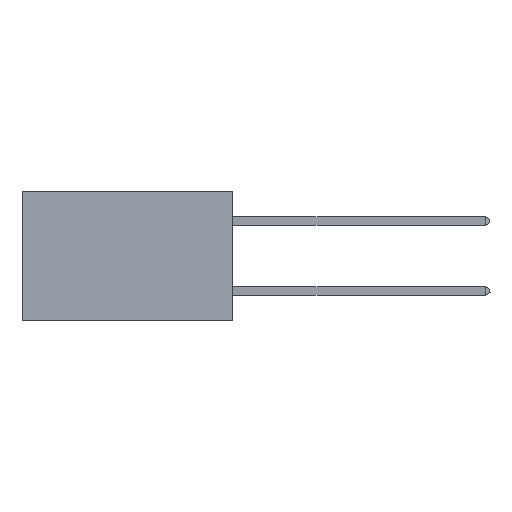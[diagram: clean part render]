
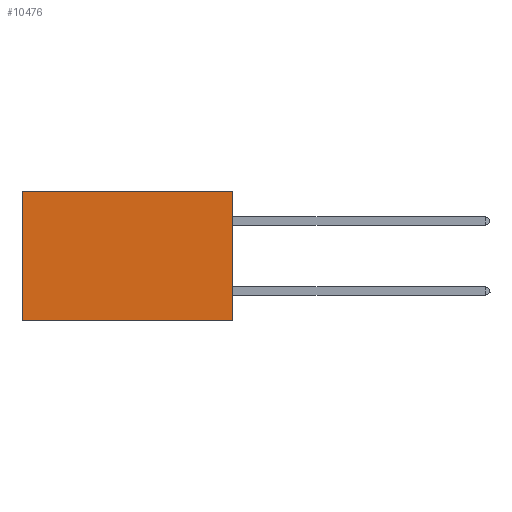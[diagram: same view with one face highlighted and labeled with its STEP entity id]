
A CAD part, left-side view. The second image highlights one B-rep face of the part: STEP entity #10476.
In plain terms, the highlighted planar face has unit normal (-1, 0, 0).
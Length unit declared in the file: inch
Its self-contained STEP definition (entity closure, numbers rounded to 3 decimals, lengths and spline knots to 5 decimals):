
#1293 = VERTEX_POINT ( 'NONE', #9393 ) ;
#2304 = LINE ( 'NONE', #4347, #10646 ) ;
#3001 = EDGE_LOOP ( 'NONE', ( #9604, #19115, #9697, #12411 ) ) ;
#3123 = LINE ( 'NONE', #4594, #8878 ) ;
#3323 = EDGE_CURVE ( 'NONE', #1293, #5030, #2304, .T. ) ;
#4347 = CARTESIAN_POINT ( 'NONE',  ( 0.2875, 0.6, 0. ) ) ;
#4439 = AXIS2_PLACEMENT_3D ( 'NONE', #18264, #18469, #19945 ) ;
#4594 = CARTESIAN_POINT ( 'NONE',  ( 0.2875, 0., 0. ) ) ;
#4647 = VERTEX_POINT ( 'NONE', #18371 ) ;
#5030 = VERTEX_POINT ( 'NONE', #10223 ) ;
#6122 = VECTOR ( 'NONE', #7002, 39.37008 ) ;
#6576 = PLANE ( 'NONE',  #4439 ) ;
#7002 = DIRECTION ( 'NONE',  ( 0., 1., 0. ) ) ;
#7457 = LINE ( 'NONE', #11922, #6122 ) ;
#8878 = VECTOR ( 'NONE', #21415, 39.37008 ) ;
#9393 = CARTESIAN_POINT ( 'NONE',  ( 0.2875, 0.6, 0. ) ) ;
#9483 = DIRECTION ( 'NONE',  ( 0., 0., -1. ) ) ;
#9604 = ORIENTED_EDGE ( 'NONE', *, *, #3323, .T. ) ;
#9697 = ORIENTED_EDGE ( 'NONE', *, *, #16907, .F. ) ;
#10223 = CARTESIAN_POINT ( 'NONE',  ( 0.2875, 0.6, -0.37 ) ) ;
#10476 = ADVANCED_FACE ( 'NONE', ( #17049 ), #6576, .F. ) ;
#10646 = VECTOR ( 'NONE', #9483, 39.37008 ) ;
#11922 = CARTESIAN_POINT ( 'NONE',  ( 0.2875, 0., -0.37 ) ) ;
#12407 = LINE ( 'NONE', #13100, #20233 ) ;
#12411 = ORIENTED_EDGE ( 'NONE', *, *, #19444, .T. ) ;
#13100 = CARTESIAN_POINT ( 'NONE',  ( 0.2875, 0., 0. ) ) ;
#13183 = DIRECTION ( 'NONE',  ( 0., 0., -1. ) ) ;
#13469 = VERTEX_POINT ( 'NONE', #16024 ) ;
#16024 = CARTESIAN_POINT ( 'NONE',  ( 0.2875, 0., 0. ) ) ;
#16636 = EDGE_CURVE ( 'NONE', #4647, #5030, #7457, .T. ) ;
#16907 = EDGE_CURVE ( 'NONE', #13469, #4647, #12407, .T. ) ;
#17049 = FACE_OUTER_BOUND ( 'NONE', #3001, .T. ) ;
#18264 = CARTESIAN_POINT ( 'NONE',  ( 0.2875, 0., 0. ) ) ;
#18371 = CARTESIAN_POINT ( 'NONE',  ( 0.2875, 0., -0.37 ) ) ;
#18469 = DIRECTION ( 'NONE',  ( 1., 0., 0. ) ) ;
#19115 = ORIENTED_EDGE ( 'NONE', *, *, #16636, .F. ) ;
#19444 = EDGE_CURVE ( 'NONE', #13469, #1293, #3123, .T. ) ;
#19945 = DIRECTION ( 'NONE',  ( 0., 0., -1. ) ) ;
#20233 = VECTOR ( 'NONE', #13183, 39.37008 ) ;
#21415 = DIRECTION ( 'NONE',  ( 0., 1., 0. ) ) ;
